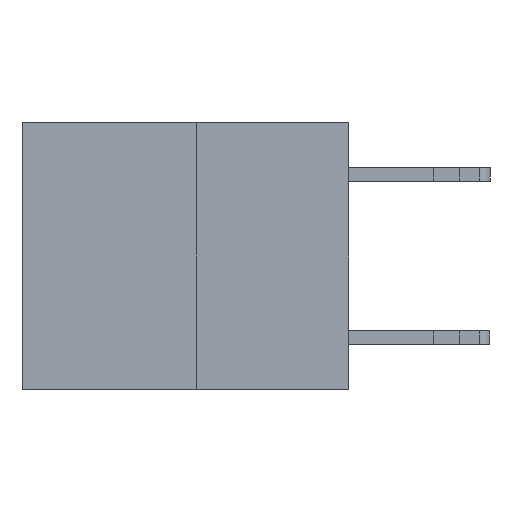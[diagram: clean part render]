
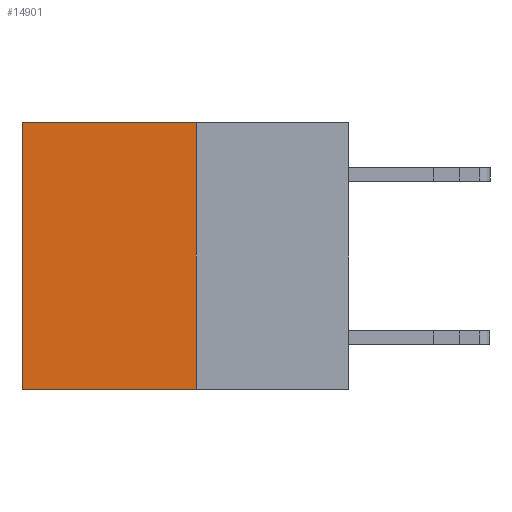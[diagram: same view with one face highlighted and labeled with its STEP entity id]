
A CAD part, left-side view. The second image highlights one B-rep face of the part: STEP entity #14901.
In plain terms, the highlighted planar face has unit normal (-1, 0, 0).
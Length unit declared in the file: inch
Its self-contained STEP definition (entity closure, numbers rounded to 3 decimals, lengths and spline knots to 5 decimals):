
#374 = CARTESIAN_POINT ( 'NONE',  ( 0.3165, 0.28, 0. ) ) ;
#1286 = LINE ( 'NONE', #4558, #14113 ) ;
#2059 = EDGE_LOOP ( 'NONE', ( #8978, #16396, #11759, #9639 ) ) ;
#2492 = DIRECTION ( 'NONE',  ( 0., 1., 0. ) ) ;
#4558 = CARTESIAN_POINT ( 'NONE',  ( 0.3165, 0.6, -0.49 ) ) ;
#5758 = PLANE ( 'NONE',  #7566 ) ;
#6117 = EDGE_CURVE ( 'NONE', #11710, #6190, #17603, .T. ) ;
#6190 = VERTEX_POINT ( 'NONE', #11002 ) ;
#6692 = EDGE_CURVE ( 'NONE', #11542, #11032, #14353, .T. ) ;
#7401 = DIRECTION ( 'NONE',  ( 0., 0., -1. ) ) ;
#7460 = DIRECTION ( 'NONE',  ( 0., 1., 0. ) ) ;
#7566 = AXIS2_PLACEMENT_3D ( 'NONE', #8524, #12997, #9929 ) ;
#7748 = VECTOR ( 'NONE', #12136, 39.37008 ) ;
#7901 = EDGE_CURVE ( 'NONE', #6190, #11032, #1286, .T. ) ;
#8524 = CARTESIAN_POINT ( 'NONE',  ( 0.3165, 0.28, -0.49 ) ) ;
#8597 = VECTOR ( 'NONE', #7460, 39.37008 ) ;
#8978 = ORIENTED_EDGE ( 'NONE', *, *, #7901, .T. ) ;
#9639 = ORIENTED_EDGE ( 'NONE', *, *, #6117, .T. ) ;
#9929 = DIRECTION ( 'NONE',  ( 0., 0., -1. ) ) ;
#10349 = CARTESIAN_POINT ( 'NONE',  ( 0.3165, 0.28, -0.49 ) ) ;
#11002 = CARTESIAN_POINT ( 'NONE',  ( 0.3165, 0.6, 0. ) ) ;
#11032 = VERTEX_POINT ( 'NONE', #16888 ) ;
#11542 = VERTEX_POINT ( 'NONE', #13525 ) ;
#11710 = VERTEX_POINT ( 'NONE', #374 ) ;
#11759 = ORIENTED_EDGE ( 'NONE', *, *, #14261, .F. ) ;
#12136 = DIRECTION ( 'NONE',  ( 0., 0., -1. ) ) ;
#12997 = DIRECTION ( 'NONE',  ( 1., 0., 0. ) ) ;
#13525 = CARTESIAN_POINT ( 'NONE',  ( 0.3165, 0.28, -0.49 ) ) ;
#14113 = VECTOR ( 'NONE', #7401, 39.37008 ) ;
#14261 = EDGE_CURVE ( 'NONE', #11710, #11542, #15254, .T. ) ;
#14353 = LINE ( 'NONE', #10349, #8597 ) ;
#14794 = VECTOR ( 'NONE', #2492, 39.37008 ) ;
#14901 = ADVANCED_FACE ( 'NONE', ( #15258 ), #5758, .F. ) ;
#14927 = CARTESIAN_POINT ( 'NONE',  ( 0.3165, 0.28, -0.49 ) ) ;
#15209 = CARTESIAN_POINT ( 'NONE',  ( 0.3165, 0.28, 0. ) ) ;
#15254 = LINE ( 'NONE', #14927, #7748 ) ;
#15258 = FACE_OUTER_BOUND ( 'NONE', #2059, .T. ) ;
#16396 = ORIENTED_EDGE ( 'NONE', *, *, #6692, .F. ) ;
#16888 = CARTESIAN_POINT ( 'NONE',  ( 0.3165, 0.6, -0.49 ) ) ;
#17603 = LINE ( 'NONE', #15209, #14794 ) ;
